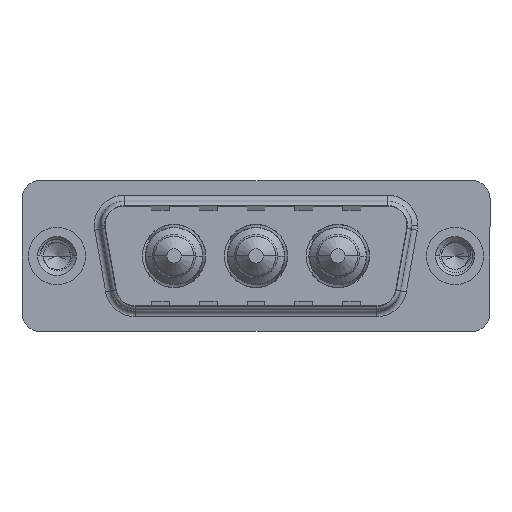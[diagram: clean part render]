
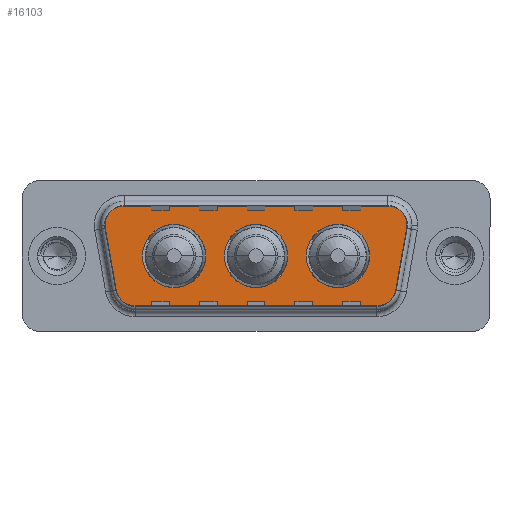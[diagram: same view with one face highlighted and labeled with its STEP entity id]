
A CAD part, top view. The second image highlights one B-rep face of the part: STEP entity #16103.
In plain terms, the highlighted planar face has unit normal (0, 0, 1).
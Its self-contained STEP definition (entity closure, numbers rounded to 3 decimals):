
#483 = ORIENTED_EDGE ( 'NONE', *, *, #15351, .T. ) ;
#566 = CARTESIAN_POINT ( 'NONE',  ( 3.441, 2.553, 0. ) ) ;
#604 = DIRECTION ( 'NONE',  ( 0., 0., 1. ) ) ;
#606 = EDGE_CURVE ( 'NONE', #11167, #6966, #14397, .T. ) ;
#638 = EDGE_CURVE ( 'NONE', #8350, #5106, #15252, .T. ) ;
#755 = EDGE_CURVE ( 'NONE', #4870, #13522, #4893, .T. ) ;
#822 = EDGE_CURVE ( 'NONE', #13522, #4870, #11584, .T. ) ;
#829 = DIRECTION ( 'NONE',  ( 1., 0., 0. ) ) ;
#852 = ORIENTED_EDGE ( 'NONE', *, *, #1452, .T. ) ;
#1292 = DIRECTION ( 'NONE',  ( 0., 0., 1. ) ) ;
#1401 = DIRECTION ( 'NONE',  ( -1., 0., 0. ) ) ;
#1452 = EDGE_CURVE ( 'NONE', #2878, #16906, #17397, .T. ) ;
#1567 = ORIENTED_EDGE ( 'NONE', *, *, #4518, .T. ) ;
#1668 = ORIENTED_EDGE ( 'NONE', *, *, #16330, .F. ) ;
#1687 = AXIS2_PLACEMENT_3D ( 'NONE', #2491, #12986, #7297 ) ;
#1737 = CIRCLE ( 'NONE', #2029, 2.65 ) ;
#1914 = VECTOR ( 'NONE', #11630, 1000. ) ;
#2029 = AXIS2_PLACEMENT_3D ( 'NONE', #9551, #1292, #10957 ) ;
#2370 = CIRCLE ( 'NONE', #4774, 2. ) ;
#2491 = CARTESIAN_POINT ( 'NONE',  ( 9.8, 0., 0. ) ) ;
#2495 = CARTESIAN_POINT ( 'NONE',  ( 27.889, 2.9, 0. ) ) ;
#2662 = AXIS2_PLACEMENT_3D ( 'NONE', #3769, #3822, #3950 ) ;
#2878 = VERTEX_POINT ( 'NONE', #15107 ) ;
#2995 = AXIS2_PLACEMENT_3D ( 'NONE', #14014, #5750, #15387 ) ;
#3223 = CARTESIAN_POINT ( 'NONE',  ( 20.85, 0., 0. ) ) ;
#3396 = EDGE_CURVE ( 'NONE', #15628, #11083, #11976, .T. ) ;
#3414 = CARTESIAN_POINT ( 'NONE',  ( 5.411, 4.9, 0. ) ) ;
#3769 = CARTESIAN_POINT ( 'NONE',  ( 27.889, 2.9, 0. ) ) ;
#3822 = DIRECTION ( 'NONE',  ( 0., 0., 1. ) ) ;
#3900 = DIRECTION ( 'NONE',  ( -1., 0., 0. ) ) ;
#3950 = DIRECTION ( 'NONE',  ( -1., 0., 0. ) ) ;
#3989 = LINE ( 'NONE', #8357, #14128 ) ;
#3996 = DIRECTION ( 'NONE',  ( 1., 0., 0. ) ) ;
#4093 = EDGE_LOOP ( 'NONE', ( #8318, #1567, #8901, #483, #852, #6341, #15863, #7292, #12177 ) ) ;
#4317 = PLANE ( 'NONE',  #2995 ) ;
#4518 = EDGE_CURVE ( 'NONE', #13234, #15628, #3989, .T. ) ;
#4735 = CARTESIAN_POINT ( 'NONE',  ( 4.464, -3.247, 0. ) ) ;
#4774 = AXIS2_PLACEMENT_3D ( 'NONE', #2495, #12142, #3900 ) ;
#4870 = VERTEX_POINT ( 'NONE', #16809 ) ;
#4893 = CIRCLE ( 'NONE', #6114, 2.65 ) ;
#4986 = VECTOR ( 'NONE', #3996, 1000. ) ;
#5003 = EDGE_CURVE ( 'NONE', #6102, #10191, #13667, .T. ) ;
#5106 = VERTEX_POINT ( 'NONE', #12523 ) ;
#5543 = EDGE_CURVE ( 'NONE', #14775, #13234, #14957, .T. ) ;
#5556 = DIRECTION ( 'NONE',  ( 0., 0., 1. ) ) ;
#5679 = VERTEX_POINT ( 'NONE', #9579 ) ;
#5750 = DIRECTION ( 'NONE',  ( 0., 0., 1. ) ) ;
#5839 = EDGE_CURVE ( 'NONE', #5106, #8350, #1737, .T. ) ;
#6102 = VERTEX_POINT ( 'NONE', #10092 ) ;
#6114 = AXIS2_PLACEMENT_3D ( 'NONE', #6992, #14907, #16162 ) ;
#6210 = CARTESIAN_POINT ( 'NONE',  ( 6.434, -2.9, 0. ) ) ;
#6341 = ORIENTED_EDGE ( 'NONE', *, *, #14618, .T. ) ;
#6627 = CARTESIAN_POINT ( 'NONE',  ( 29.889, 2.9, 0. ) ) ;
#6880 = CARTESIAN_POINT ( 'NONE',  ( 28.836, -3.247, 0. ) ) ;
#6966 = VERTEX_POINT ( 'NONE', #8298 ) ;
#6992 = CARTESIAN_POINT ( 'NONE',  ( 9.8, 0., 0. ) ) ;
#7044 = CARTESIAN_POINT ( 'NONE',  ( 5.411, 2.9, 0. ) ) ;
#7292 = ORIENTED_EDGE ( 'NONE', *, *, #606, .T. ) ;
#7297 = DIRECTION ( 'NONE',  ( 1., 0., 0. ) ) ;
#7641 = EDGE_LOOP ( 'NONE', ( #16164, #15250 ) ) ;
#8298 = CARTESIAN_POINT ( 'NONE',  ( 6.434, -4.9, 0. ) ) ;
#8318 = ORIENTED_EDGE ( 'NONE', *, *, #5543, .T. ) ;
#8350 = VERTEX_POINT ( 'NONE', #3223 ) ;
#8357 = CARTESIAN_POINT ( 'NONE',  ( 29.859, 2.553, 0. ) ) ;
#8401 = DIRECTION ( 'NONE',  ( 1., 0., 0. ) ) ;
#8528 = DIRECTION ( 'NONE',  ( 0., 0., 1. ) ) ;
#8543 = CARTESIAN_POINT ( 'NONE',  ( 29.859, 2.553, 0. ) ) ;
#8596 = LINE ( 'NONE', #13697, #4986 ) ;
#8841 = CARTESIAN_POINT ( 'NONE',  ( 16.65, 0., 0. ) ) ;
#8901 = ORIENTED_EDGE ( 'NONE', *, *, #3396, .T. ) ;
#8935 = EDGE_LOOP ( 'NONE', ( #1668, #10214 ) ) ;
#9004 = FACE_BOUND ( 'NONE', #9599, .T. ) ;
#9082 = DIRECTION ( 'NONE',  ( 0., 0., 1. ) ) ;
#9551 = CARTESIAN_POINT ( 'NONE',  ( 23.5, 0., 0. ) ) ;
#9560 = EDGE_CURVE ( 'NONE', #6966, #14775, #8596, .T. ) ;
#9579 = CARTESIAN_POINT ( 'NONE',  ( 3.441, 2.553, 0. ) ) ;
#9599 = EDGE_LOOP ( 'NONE', ( #11058, #10508 ) ) ;
#9849 = EDGE_CURVE ( 'NONE', #5679, #11167, #12960, .T. ) ;
#10092 = CARTESIAN_POINT ( 'NONE',  ( 14., 0., 0. ) ) ;
#10093 = CIRCLE ( 'NONE', #14090, 2.65 ) ;
#10191 = VERTEX_POINT ( 'NONE', #16487 ) ;
#10214 = ORIENTED_EDGE ( 'NONE', *, *, #5003, .F. ) ;
#10221 = DIRECTION ( 'NONE',  ( 0., 0., 1. ) ) ;
#10267 = DIRECTION ( 'NONE',  ( 1., 0., 0. ) ) ;
#10285 = CARTESIAN_POINT ( 'NONE',  ( 23.5, 0., 0. ) ) ;
#10318 = CIRCLE ( 'NONE', #14106, 2. ) ;
#10508 = ORIENTED_EDGE ( 'NONE', *, *, #638, .F. ) ;
#10957 = DIRECTION ( 'NONE',  ( 1., 0., 0. ) ) ;
#11058 = ORIENTED_EDGE ( 'NONE', *, *, #5839, .F. ) ;
#11083 = VERTEX_POINT ( 'NONE', #6627 ) ;
#11167 = VERTEX_POINT ( 'NONE', #4735 ) ;
#11438 = CARTESIAN_POINT ( 'NONE',  ( 26.866, -4.9, 0. ) ) ;
#11584 = CIRCLE ( 'NONE', #1687, 2.65 ) ;
#11630 = DIRECTION ( 'NONE',  ( 0.174, -0.985, 0. ) ) ;
#11827 = CARTESIAN_POINT ( 'NONE',  ( 12.45, 0., 0. ) ) ;
#11976 = CIRCLE ( 'NONE', #2662, 2. ) ;
#12142 = DIRECTION ( 'NONE',  ( 0., 0., 1. ) ) ;
#12177 = ORIENTED_EDGE ( 'NONE', *, *, #9560, .T. ) ;
#12283 = FACE_OUTER_BOUND ( 'NONE', #4093, .T. ) ;
#12322 = AXIS2_PLACEMENT_3D ( 'NONE', #13807, #5556, #15188 ) ;
#12523 = CARTESIAN_POINT ( 'NONE',  ( 26.15, 0., 0. ) ) ;
#12886 = VECTOR ( 'NONE', #1401, 1000. ) ;
#12960 = LINE ( 'NONE', #566, #1914 ) ;
#12986 = DIRECTION ( 'NONE',  ( 0., 0., 1. ) ) ;
#13234 = VERTEX_POINT ( 'NONE', #6880 ) ;
#13522 = VERTEX_POINT ( 'NONE', #11827 ) ;
#13667 = CIRCLE ( 'NONE', #12322, 2.65 ) ;
#13697 = CARTESIAN_POINT ( 'NONE',  ( 6.434, -4.9, 0. ) ) ;
#13807 = CARTESIAN_POINT ( 'NONE',  ( 16.65, 0., 0. ) ) ;
#14014 = CARTESIAN_POINT ( 'NONE',  ( 26.866, -2.9, 0. ) ) ;
#14090 = AXIS2_PLACEMENT_3D ( 'NONE', #8841, #604, #10267 ) ;
#14106 = AXIS2_PLACEMENT_3D ( 'NONE', #7044, #16677, #8401 ) ;
#14128 = VECTOR ( 'NONE', #16393, 1000. ) ;
#14397 = CIRCLE ( 'NONE', #16608, 2. ) ;
#14618 = EDGE_CURVE ( 'NONE', #16906, #5679, #10318, .T. ) ;
#14775 = VERTEX_POINT ( 'NONE', #11438 ) ;
#14853 = DIRECTION ( 'NONE',  ( -1., 0., 0. ) ) ;
#14907 = DIRECTION ( 'NONE',  ( 0., 0., 1. ) ) ;
#14957 = CIRCLE ( 'NONE', #17524, 2. ) ;
#15107 = CARTESIAN_POINT ( 'NONE',  ( 27.889, 4.9, 0. ) ) ;
#15188 = DIRECTION ( 'NONE',  ( 1., 0., 0. ) ) ;
#15250 = ORIENTED_EDGE ( 'NONE', *, *, #755, .F. ) ;
#15252 = CIRCLE ( 'NONE', #15711, 2.65 ) ;
#15351 = EDGE_CURVE ( 'NONE', #11083, #2878, #2370, .T. ) ;
#15387 = DIRECTION ( 'NONE',  ( 1., 0., 0. ) ) ;
#15628 = VERTEX_POINT ( 'NONE', #8543 ) ;
#15677 = CARTESIAN_POINT ( 'NONE',  ( 5.411, 4.9, 0. ) ) ;
#15711 = AXIS2_PLACEMENT_3D ( 'NONE', #10285, #10221, #16754 ) ;
#15863 = ORIENTED_EDGE ( 'NONE', *, *, #9849, .T. ) ;
#15959 = FACE_BOUND ( 'NONE', #7641, .T. ) ;
#16103 = ADVANCED_FACE ( 'NONE', ( #16371, #9004, #15959, #12283 ), #4317, .T. ) ;
#16162 = DIRECTION ( 'NONE',  ( 1., 0., 0. ) ) ;
#16164 = ORIENTED_EDGE ( 'NONE', *, *, #822, .F. ) ;
#16330 = EDGE_CURVE ( 'NONE', #10191, #6102, #10093, .T. ) ;
#16371 = FACE_BOUND ( 'NONE', #8935, .T. ) ;
#16393 = DIRECTION ( 'NONE',  ( 0.174, 0.985, 0. ) ) ;
#16487 = CARTESIAN_POINT ( 'NONE',  ( 19.3, 0., 0. ) ) ;
#16608 = AXIS2_PLACEMENT_3D ( 'NONE', #6210, #8528, #14853 ) ;
#16677 = DIRECTION ( 'NONE',  ( 0., 0., 1. ) ) ;
#16754 = DIRECTION ( 'NONE',  ( 1., 0., 0. ) ) ;
#16809 = CARTESIAN_POINT ( 'NONE',  ( 7.15, 0., 0. ) ) ;
#16906 = VERTEX_POINT ( 'NONE', #3414 ) ;
#17390 = CARTESIAN_POINT ( 'NONE',  ( 26.866, -2.9, 0. ) ) ;
#17397 = LINE ( 'NONE', #15677, #12886 ) ;
#17524 = AXIS2_PLACEMENT_3D ( 'NONE', #17390, #9082, #829 ) ;
